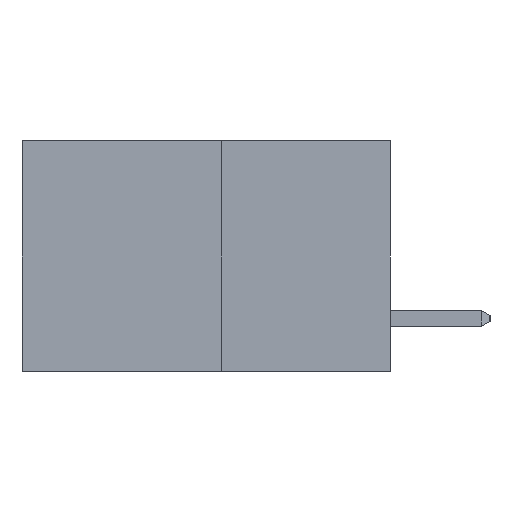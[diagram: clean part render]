
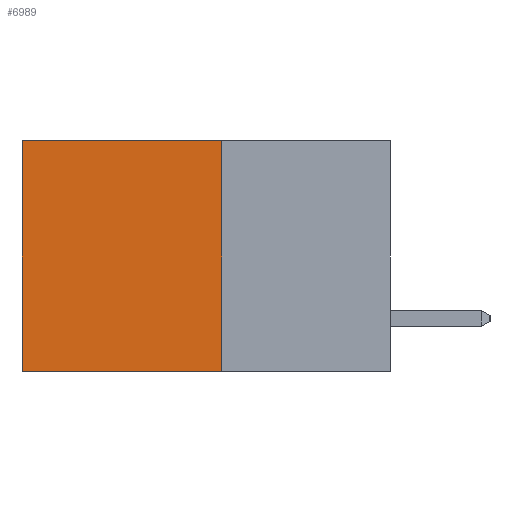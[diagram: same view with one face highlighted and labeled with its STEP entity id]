
A CAD part, left-side view. The second image highlights one B-rep face of the part: STEP entity #6989.
In plain terms, the highlighted planar face has unit normal (-1, 0, 0).
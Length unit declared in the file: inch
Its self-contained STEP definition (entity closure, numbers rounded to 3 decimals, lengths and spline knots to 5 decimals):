
#937 = ORIENTED_EDGE ( 'NONE', *, *, #16105, .T. ) ;
#2276 = VECTOR ( 'NONE', #8218, 39.37008 ) ;
#2731 = VERTEX_POINT ( 'NONE', #15772 ) ;
#2900 = VERTEX_POINT ( 'NONE', #6490 ) ;
#4319 = FACE_OUTER_BOUND ( 'NONE', #20139, .T. ) ;
#5310 = ORIENTED_EDGE ( 'NONE', *, *, #21118, .F. ) ;
#6490 = CARTESIAN_POINT ( 'NONE',  ( 0.277, 0.59, 0. ) ) ;
#6914 = CARTESIAN_POINT ( 'NONE',  ( 0.277, 0.27, -0.37 ) ) ;
#6989 = ADVANCED_FACE ( 'NONE', ( #4319 ), #19704, .F. ) ;
#8218 = DIRECTION ( 'NONE',  ( 0., 1., 0. ) ) ;
#8954 = VECTOR ( 'NONE', #20493, 39.37008 ) ;
#9160 = AXIS2_PLACEMENT_3D ( 'NONE', #19733, #14596, #14569 ) ;
#10192 = DIRECTION ( 'NONE',  ( 0., 0., -1. ) ) ;
#11511 = CARTESIAN_POINT ( 'NONE',  ( 0.277, 0.27, 0. ) ) ;
#11807 = CARTESIAN_POINT ( 'NONE',  ( 0.277, 0.27, -0.37 ) ) ;
#12389 = CARTESIAN_POINT ( 'NONE',  ( 0.277, 0.59, -0.37 ) ) ;
#12712 = VERTEX_POINT ( 'NONE', #17897 ) ;
#12840 = ORIENTED_EDGE ( 'NONE', *, *, #16414, .T. ) ;
#13028 = VECTOR ( 'NONE', #19007, 39.37008 ) ;
#13311 = LINE ( 'NONE', #12389, #8954 ) ;
#14241 = LINE ( 'NONE', #6914, #18097 ) ;
#14569 = DIRECTION ( 'NONE',  ( 0., 0., -1. ) ) ;
#14596 = DIRECTION ( 'NONE',  ( 1., 0., 0. ) ) ;
#15442 = ORIENTED_EDGE ( 'NONE', *, *, #17420, .F. ) ;
#15713 = CARTESIAN_POINT ( 'NONE',  ( 0.277, 0.27, -0.37 ) ) ;
#15772 = CARTESIAN_POINT ( 'NONE',  ( 0.277, 0.27, 0. ) ) ;
#15881 = VERTEX_POINT ( 'NONE', #11807 ) ;
#16105 = EDGE_CURVE ( 'NONE', #2900, #12712, #13311, .T. ) ;
#16414 = EDGE_CURVE ( 'NONE', #2731, #2900, #20168, .T. ) ;
#17393 = LINE ( 'NONE', #15713, #13028 ) ;
#17420 = EDGE_CURVE ( 'NONE', #15881, #12712, #17393, .T. ) ;
#17897 = CARTESIAN_POINT ( 'NONE',  ( 0.277, 0.59, -0.37 ) ) ;
#18097 = VECTOR ( 'NONE', #10192, 39.37008 ) ;
#19007 = DIRECTION ( 'NONE',  ( 0., 1., 0. ) ) ;
#19704 = PLANE ( 'NONE',  #9160 ) ;
#19733 = CARTESIAN_POINT ( 'NONE',  ( 0.277, 0.27, -0.37 ) ) ;
#20139 = EDGE_LOOP ( 'NONE', ( #937, #15442, #5310, #12840 ) ) ;
#20168 = LINE ( 'NONE', #11511, #2276 ) ;
#20493 = DIRECTION ( 'NONE',  ( 0., 0., -1. ) ) ;
#21118 = EDGE_CURVE ( 'NONE', #2731, #15881, #14241, .T. ) ;
